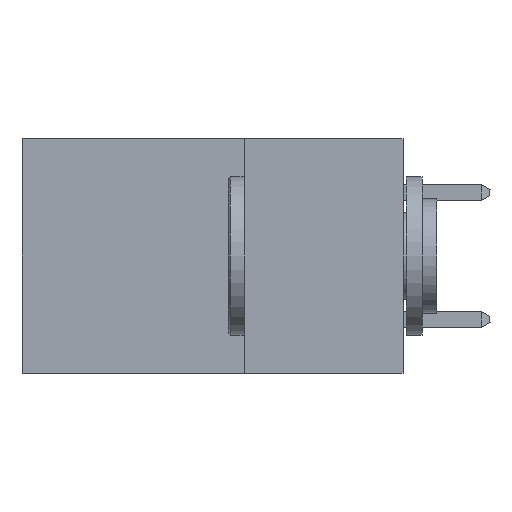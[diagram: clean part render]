
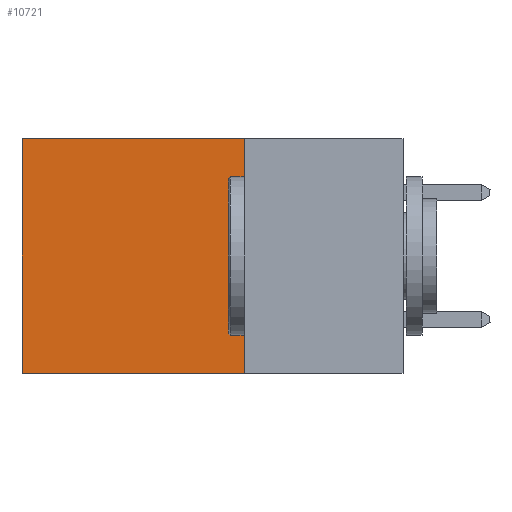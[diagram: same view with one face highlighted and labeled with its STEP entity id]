
A CAD part, left-side view. The second image highlights one B-rep face of the part: STEP entity #10721.
In plain terms, the highlighted planar face has unit normal (-1, 0, 0).
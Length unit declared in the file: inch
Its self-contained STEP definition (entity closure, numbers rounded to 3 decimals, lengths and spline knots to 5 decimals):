
#383 = CARTESIAN_POINT ( 'NONE',  ( 0.2875, 0.6, 0. ) ) ;
#441 = EDGE_CURVE ( 'NONE', #3539, #7536, #1372, .T. ) ;
#1021 = CARTESIAN_POINT ( 'NONE',  ( 0.2875, 0.25, 0. ) ) ;
#1042 = CARTESIAN_POINT ( 'NONE',  ( 0.2875, 0.6, -0.37 ) ) ;
#1090 = CARTESIAN_POINT ( 'NONE',  ( 0.2875, 0.25, -0.37 ) ) ;
#1254 = VECTOR ( 'NONE', #4168, 39.37008 ) ;
#1372 = LINE ( 'NONE', #2890, #3365 ) ;
#1518 = DIRECTION ( 'NONE',  ( 0., 1., 0. ) ) ;
#2228 = LINE ( 'NONE', #1021, #11762 ) ;
#2890 = CARTESIAN_POINT ( 'NONE',  ( 0.2875, 0.25, 0. ) ) ;
#3076 = ORIENTED_EDGE ( 'NONE', *, *, #8217, .T. ) ;
#3119 = VERTEX_POINT ( 'NONE', #1090 ) ;
#3365 = VECTOR ( 'NONE', #4989, 39.37008 ) ;
#3429 = FACE_OUTER_BOUND ( 'NONE', #6438, .T. ) ;
#3539 = VERTEX_POINT ( 'NONE', #10598 ) ;
#3948 = DIRECTION ( 'NONE',  ( 0., 0., -1. ) ) ;
#4168 = DIRECTION ( 'NONE',  ( 0., 0., -1. ) ) ;
#4665 = PLANE ( 'NONE',  #6129 ) ;
#4989 = DIRECTION ( 'NONE',  ( 0., 1., 0. ) ) ;
#5602 = DIRECTION ( 'NONE',  ( 1., 0., 0. ) ) ;
#5862 = ORIENTED_EDGE ( 'NONE', *, *, #6567, .F. ) ;
#6081 = VECTOR ( 'NONE', #1518, 39.37008 ) ;
#6129 = AXIS2_PLACEMENT_3D ( 'NONE', #11050, #5602, #11970 ) ;
#6438 = EDGE_LOOP ( 'NONE', ( #3076, #10411, #5862, #8305 ) ) ;
#6567 = EDGE_CURVE ( 'NONE', #3539, #3119, #2228, .T. ) ;
#7189 = CARTESIAN_POINT ( 'NONE',  ( 0.2875, 0.25, -0.37 ) ) ;
#7536 = VERTEX_POINT ( 'NONE', #383 ) ;
#7941 = LINE ( 'NONE', #7189, #6081 ) ;
#8217 = EDGE_CURVE ( 'NONE', #7536, #10855, #9066, .T. ) ;
#8305 = ORIENTED_EDGE ( 'NONE', *, *, #441, .T. ) ;
#9066 = LINE ( 'NONE', #11489, #1254 ) ;
#9398 = EDGE_CURVE ( 'NONE', #3119, #10855, #7941, .T. ) ;
#10411 = ORIENTED_EDGE ( 'NONE', *, *, #9398, .F. ) ;
#10598 = CARTESIAN_POINT ( 'NONE',  ( 0.2875, 0.25, 0. ) ) ;
#10721 = ADVANCED_FACE ( 'NONE', ( #3429 ), #4665, .F. ) ;
#10855 = VERTEX_POINT ( 'NONE', #1042 ) ;
#11050 = CARTESIAN_POINT ( 'NONE',  ( 0.2875, 0.25, 0. ) ) ;
#11489 = CARTESIAN_POINT ( 'NONE',  ( 0.2875, 0.6, 0. ) ) ;
#11762 = VECTOR ( 'NONE', #3948, 39.37008 ) ;
#11970 = DIRECTION ( 'NONE',  ( 0., 0., -1. ) ) ;
